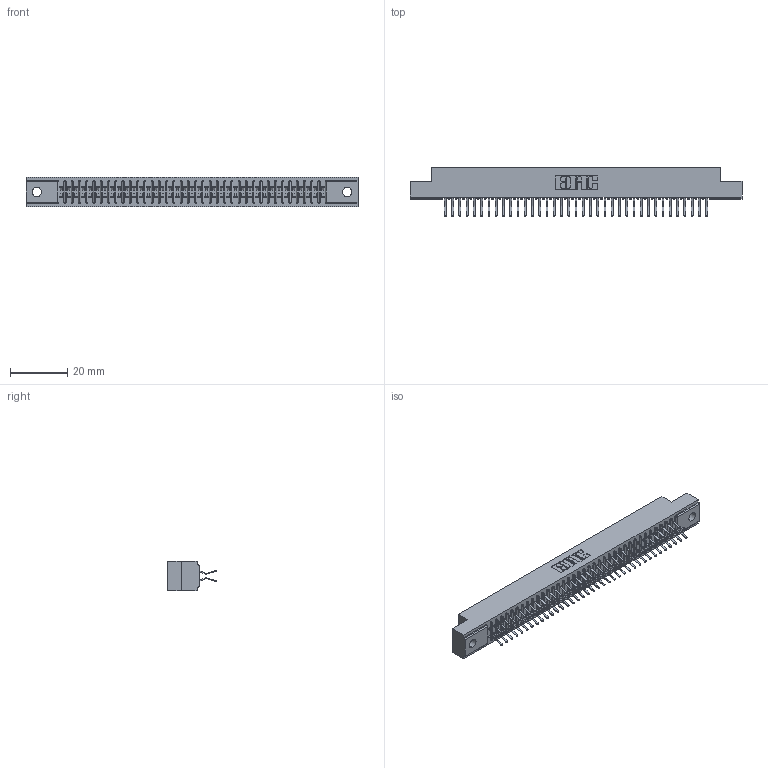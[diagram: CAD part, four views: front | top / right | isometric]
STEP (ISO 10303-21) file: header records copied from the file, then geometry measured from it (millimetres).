
FILE_DESCRIPTION (( 'STEP AP203' ), '1' );
FILE_NAME ('391-074-556-202.STEP', '2018-08-09T14:47:16', ( '' ), ( '' ), 'SwSTEP 2.0', 'SolidWorks 2016', '' );
FILE_SCHEMA (( 'CONFIG_CONTROL_DESIGN' ));
Length unit declared in the file: inch
Products named in the file (3): 341 Part_.128 (3.25) Dia Mounting Holes; 341-292-001_341-292-156; 391-074-556-202
Assembly tree (75 placements, depth 2):
  391-074-556-202
    341 Part_.128 (3.25) Dia Mounting Holes
    341-292-001_341-292-156  x74
Bounding box: 116.2 x 17.07 x 10.16 mm (x, y, z)
Volume: 8560.2 mm3; surface area: 14963.7 mm2
Topology: 75 solids, 75 shells, 5296 faces, 15375 edges, 9974 vertices
Faces by surface type: plane 3028, cylinder 2120, sphere 76, torus 72
Entity records: 45586 total; most frequent: CARTESIAN_POINT 7579, ORIENTED_EDGE 7530, DIRECTION 7363, EDGE_CURVE 3765, LINE 3031, VECTOR 3031, VERTEX_POINT 2382, AXIS2_PLACEMENT_3D 2166
